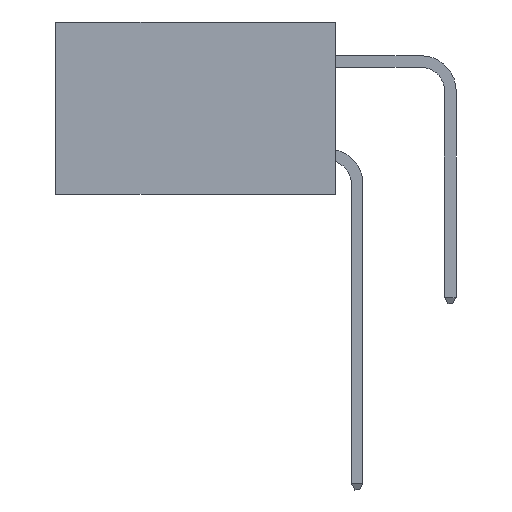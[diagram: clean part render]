
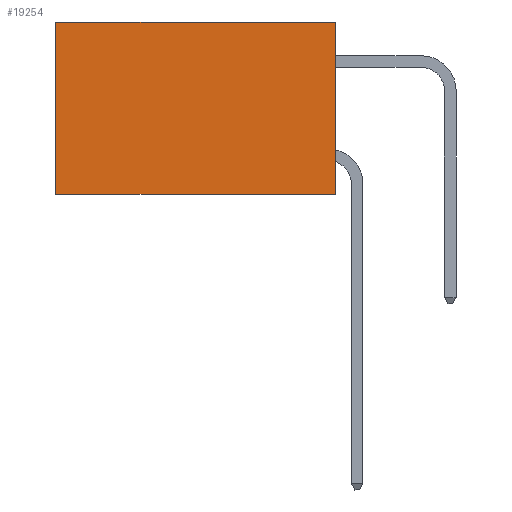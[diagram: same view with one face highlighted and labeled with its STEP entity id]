
A CAD part, left-side view. The second image highlights one B-rep face of the part: STEP entity #19254.
In plain terms, the highlighted planar face has unit normal (-1, 0, 0).
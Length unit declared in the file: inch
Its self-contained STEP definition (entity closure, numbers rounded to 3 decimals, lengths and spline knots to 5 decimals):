
#73 = VECTOR ( 'NONE', #3273, 39.37008 ) ;
#903 = CARTESIAN_POINT ( 'NONE',  ( 0.2875, 0., 0. ) ) ;
#1321 = ORIENTED_EDGE ( 'NONE', *, *, #22563, .T. ) ;
#1904 = PLANE ( 'NONE',  #27094 ) ;
#3273 = DIRECTION ( 'NONE',  ( 0., 0., -1. ) ) ;
#4179 = CARTESIAN_POINT ( 'NONE',  ( 0.2875, 0., 0. ) ) ;
#4313 = ORIENTED_EDGE ( 'NONE', *, *, #26332, .F. ) ;
#5004 = LINE ( 'NONE', #25783, #28200 ) ;
#5844 = VERTEX_POINT ( 'NONE', #22031 ) ;
#6487 = CARTESIAN_POINT ( 'NONE',  ( 0.2875, 0., 0. ) ) ;
#8752 = DIRECTION ( 'NONE',  ( 0., 0., -1. ) ) ;
#9844 = ORIENTED_EDGE ( 'NONE', *, *, #25643, .F. ) ;
#11934 = FACE_OUTER_BOUND ( 'NONE', #16920, .T. ) ;
#12352 = DIRECTION ( 'NONE',  ( 0., 1., 0. ) ) ;
#12462 = CARTESIAN_POINT ( 'NONE',  ( 0.2875, 0.6, 0. ) ) ;
#13356 = CARTESIAN_POINT ( 'NONE',  ( 0.2875, 0.6, 0. ) ) ;
#13845 = VECTOR ( 'NONE', #14714, 39.37008 ) ;
#13925 = CARTESIAN_POINT ( 'NONE',  ( 0.2875, 0.6, -0.37 ) ) ;
#14714 = DIRECTION ( 'NONE',  ( 0., 0., -1. ) ) ;
#16536 = EDGE_CURVE ( 'NONE', #27455, #18262, #19793, .T. ) ;
#16920 = EDGE_LOOP ( 'NONE', ( #25241, #4313, #9844, #1321 ) ) ;
#18262 = VERTEX_POINT ( 'NONE', #13925 ) ;
#18897 = VERTEX_POINT ( 'NONE', #20953 ) ;
#19254 = ADVANCED_FACE ( 'NONE', ( #11934 ), #1904, .F. ) ;
#19793 = LINE ( 'NONE', #12462, #13845 ) ;
#20402 = LINE ( 'NONE', #4179, #25642 ) ;
#20953 = CARTESIAN_POINT ( 'NONE',  ( 0.2875, 0., 0. ) ) ;
#22031 = CARTESIAN_POINT ( 'NONE',  ( 0.2875, 0., -0.37 ) ) ;
#22193 = DIRECTION ( 'NONE',  ( 0., 1., 0. ) ) ;
#22203 = DIRECTION ( 'NONE',  ( 1., 0., 0. ) ) ;
#22563 = EDGE_CURVE ( 'NONE', #18897, #27455, #20402, .T. ) ;
#23344 = LINE ( 'NONE', #903, #73 ) ;
#25241 = ORIENTED_EDGE ( 'NONE', *, *, #16536, .T. ) ;
#25642 = VECTOR ( 'NONE', #22193, 39.37008 ) ;
#25643 = EDGE_CURVE ( 'NONE', #18897, #5844, #23344, .T. ) ;
#25783 = CARTESIAN_POINT ( 'NONE',  ( 0.2875, 0., -0.37 ) ) ;
#26332 = EDGE_CURVE ( 'NONE', #5844, #18262, #5004, .T. ) ;
#27094 = AXIS2_PLACEMENT_3D ( 'NONE', #6487, #22203, #8752 ) ;
#27455 = VERTEX_POINT ( 'NONE', #13356 ) ;
#28200 = VECTOR ( 'NONE', #12352, 39.37008 ) ;
